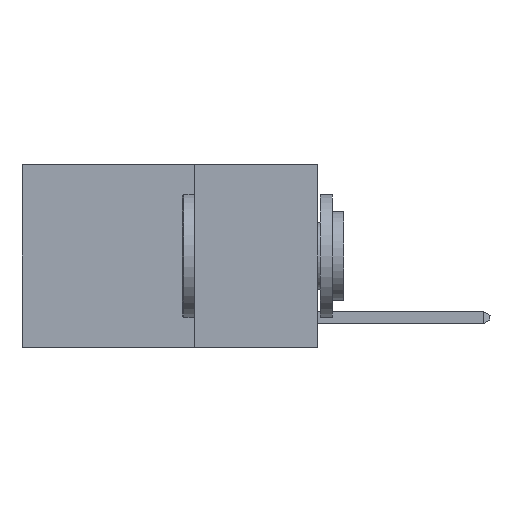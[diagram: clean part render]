
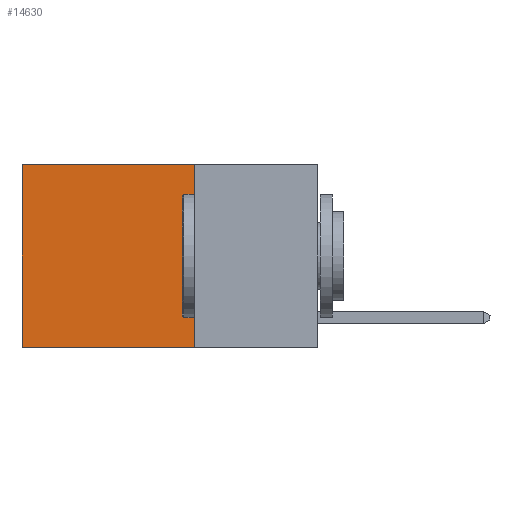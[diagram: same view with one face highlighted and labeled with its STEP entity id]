
A CAD part, left-side view. The second image highlights one B-rep face of the part: STEP entity #14630.
In plain terms, the highlighted planar face has unit normal (-1, 0, 0).
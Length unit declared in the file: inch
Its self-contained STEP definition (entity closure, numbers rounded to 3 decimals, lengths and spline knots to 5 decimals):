
#582 = CARTESIAN_POINT ( 'NONE',  ( 0.2625, 0.6, 0. ) ) ;
#1077 = ORIENTED_EDGE ( 'NONE', *, *, #4482, .T. ) ;
#1325 = EDGE_CURVE ( 'NONE', #11210, #11562, #14777, .T. ) ;
#1795 = CARTESIAN_POINT ( 'NONE',  ( 0.2625, 0.25, 0. ) ) ;
#1872 = VECTOR ( 'NONE', #7864, 39.37008 ) ;
#2270 = EDGE_CURVE ( 'NONE', #2437, #11562, #3831, .T. ) ;
#2437 = VERTEX_POINT ( 'NONE', #3647 ) ;
#2921 = ORIENTED_EDGE ( 'NONE', *, *, #1325, .T. ) ;
#3647 = CARTESIAN_POINT ( 'NONE',  ( 0.2625, 0.25, -0.37 ) ) ;
#3831 = LINE ( 'NONE', #14201, #10704 ) ;
#4371 = CARTESIAN_POINT ( 'NONE',  ( 0.2625, 0.25, 0. ) ) ;
#4398 = DIRECTION ( 'NONE',  ( 0., 1., 0. ) ) ;
#4404 = CARTESIAN_POINT ( 'NONE',  ( 0.2625, 0.6, 0. ) ) ;
#4482 = EDGE_CURVE ( 'NONE', #8966, #11210, #7892, .T. ) ;
#5032 = ORIENTED_EDGE ( 'NONE', *, *, #13555, .F. ) ;
#6711 = DIRECTION ( 'NONE',  ( 1., 0., 0. ) ) ;
#7162 = CARTESIAN_POINT ( 'NONE',  ( 0.2625, 0.25, 0. ) ) ;
#7864 = DIRECTION ( 'NONE',  ( 0., 0., -1. ) ) ;
#7892 = LINE ( 'NONE', #1795, #10702 ) ;
#8966 = VERTEX_POINT ( 'NONE', #7162 ) ;
#9782 = CARTESIAN_POINT ( 'NONE',  ( 0.2625, 0.6, -0.37 ) ) ;
#10036 = FACE_OUTER_BOUND ( 'NONE', #11892, .T. ) ;
#10702 = VECTOR ( 'NONE', #4398, 39.37008 ) ;
#10704 = VECTOR ( 'NONE', #14344, 39.37008 ) ;
#11210 = VERTEX_POINT ( 'NONE', #582 ) ;
#11240 = PLANE ( 'NONE',  #11309 ) ;
#11309 = AXIS2_PLACEMENT_3D ( 'NONE', #13360, #6711, #14651 ) ;
#11562 = VERTEX_POINT ( 'NONE', #9782 ) ;
#11892 = EDGE_LOOP ( 'NONE', ( #2921, #14303, #5032, #1077 ) ) ;
#13360 = CARTESIAN_POINT ( 'NONE',  ( 0.2625, 0.25, 0. ) ) ;
#13444 = VECTOR ( 'NONE', #13710, 39.37008 ) ;
#13555 = EDGE_CURVE ( 'NONE', #8966, #2437, #13816, .T. ) ;
#13710 = DIRECTION ( 'NONE',  ( 0., 0., -1. ) ) ;
#13816 = LINE ( 'NONE', #4371, #1872 ) ;
#14201 = CARTESIAN_POINT ( 'NONE',  ( 0.2625, 0.25, -0.37 ) ) ;
#14303 = ORIENTED_EDGE ( 'NONE', *, *, #2270, .F. ) ;
#14344 = DIRECTION ( 'NONE',  ( 0., 1., 0. ) ) ;
#14630 = ADVANCED_FACE ( 'NONE', ( #10036 ), #11240, .F. ) ;
#14651 = DIRECTION ( 'NONE',  ( 0., 0., -1. ) ) ;
#14777 = LINE ( 'NONE', #4404, #13444 ) ;
